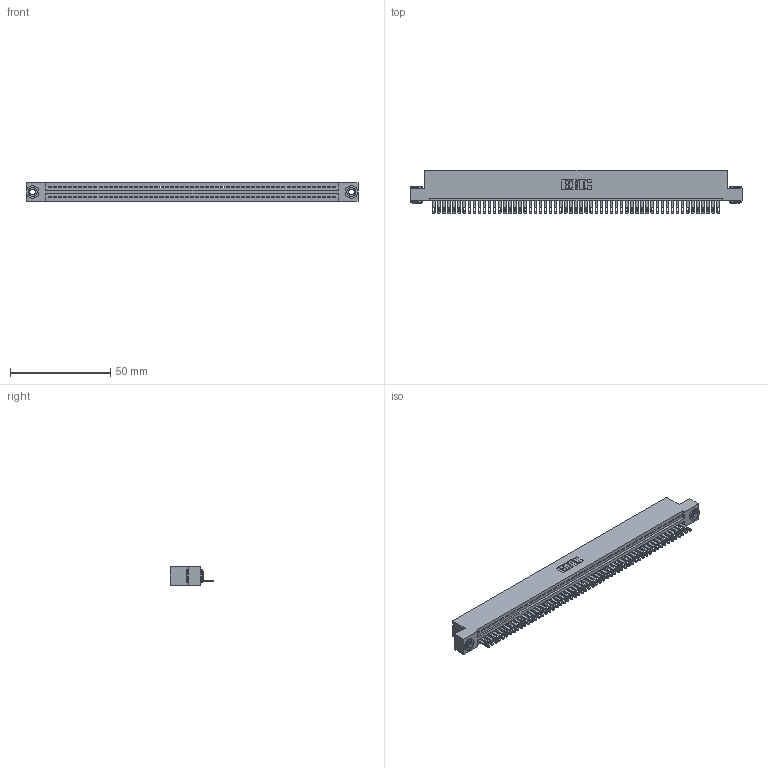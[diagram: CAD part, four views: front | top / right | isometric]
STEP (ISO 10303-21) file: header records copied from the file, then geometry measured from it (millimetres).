
FILE_DESCRIPTION (( 'STEP AP203' ), '1' );
FILE_NAME ('895-057-500-103.STEP', '2020-09-27T17:08:02', ( '' ), ( '' ), 'SwSTEP 2.0', 'SolidWorks 2020', '' );
FILE_SCHEMA (( 'CONFIG_CONTROL_DESIGN' ));
Length unit declared in the file: inch
Products named in the file (4): 345-250-002_345-250-002-102; 845 Part_Flush Mounting Lugs - 0.156 Dia-TH; 895-057-500-103; 345-292-001_345-293-100
Assembly tree (60 placements, depth 2):
  895-057-500-103
    845 Part_Flush Mounting Lugs - 0.156 Dia-TH
    345-292-001_345-293-100  x57
    345-250-002_345-250-002-102  x2
Bounding box: 165.99 x 21.51 x 9.4 mm (x, y, z)
Volume: 15943.4 mm3; surface area: 21733.6 mm2
Topology: 60 solids, 60 shells, 3242 faces, 9993 edges, 6658 vertices
Faces by surface type: plane 2028, cylinder 1206, cone 8
Entity records: 41460 total; most frequent: CARTESIAN_POINT 7158, ORIENTED_EDGE 7142, DIRECTION 6263, EDGE_CURVE 3571, VECTOR 3183, LINE 3183, VERTEX_POINT 2378, AXIS2_PLACEMENT_3D 1540
